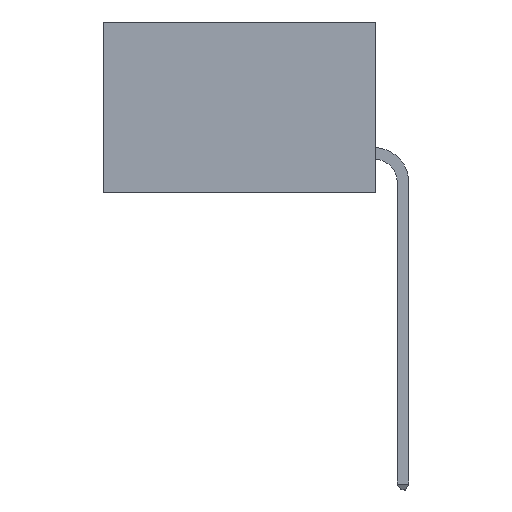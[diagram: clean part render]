
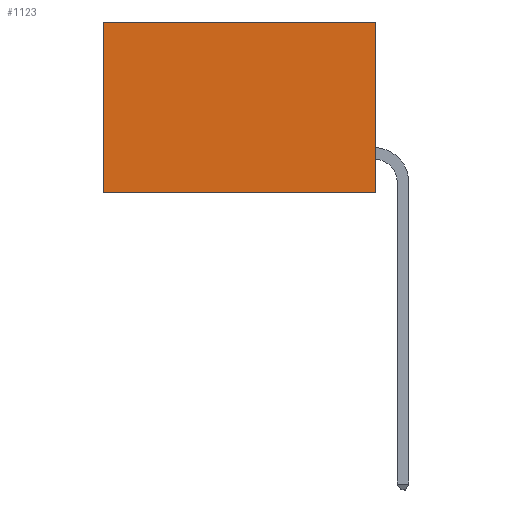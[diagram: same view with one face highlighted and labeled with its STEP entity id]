
A CAD part, left-side view. The second image highlights one B-rep face of the part: STEP entity #1123.
In plain terms, the highlighted planar face has unit normal (-1, 0, 0).
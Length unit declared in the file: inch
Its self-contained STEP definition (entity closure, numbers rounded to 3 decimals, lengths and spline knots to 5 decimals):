
#225 = CARTESIAN_POINT ( 'NONE',  ( 0.277, 0., -0.37 ) ) ;
#475 = VECTOR ( 'NONE', #12674, 39.37008 ) ;
#764 = AXIS2_PLACEMENT_3D ( 'NONE', #2841, #3631, #5499 ) ;
#955 = DIRECTION ( 'NONE',  ( 0., 1., 0. ) ) ;
#1123 = ADVANCED_FACE ( 'NONE', ( #13194 ), #10374, .F. ) ;
#1459 = VERTEX_POINT ( 'NONE', #225 ) ;
#1696 = VECTOR ( 'NONE', #955, 39.37008 ) ;
#2172 = EDGE_CURVE ( 'NONE', #10078, #1459, #9218, .T. ) ;
#2841 = CARTESIAN_POINT ( 'NONE',  ( 0.277, 0., -0.37 ) ) ;
#3599 = ORIENTED_EDGE ( 'NONE', *, *, #5665, .T. ) ;
#3601 = CARTESIAN_POINT ( 'NONE',  ( 0.277, 0., -0.37 ) ) ;
#3631 = DIRECTION ( 'NONE',  ( 1., 0., 0. ) ) ;
#3669 = ORIENTED_EDGE ( 'NONE', *, *, #4193, .F. ) ;
#3765 = ORIENTED_EDGE ( 'NONE', *, *, #2172, .F. ) ;
#3776 = ORIENTED_EDGE ( 'NONE', *, *, #13361, .T. ) ;
#4193 = EDGE_CURVE ( 'NONE', #1459, #6478, #6012, .T. ) ;
#5122 = VECTOR ( 'NONE', #7197, 39.37008 ) ;
#5499 = DIRECTION ( 'NONE',  ( 0., 0., -1. ) ) ;
#5665 = EDGE_CURVE ( 'NONE', #6463, #6478, #8031, .T. ) ;
#6012 = LINE ( 'NONE', #3601, #11280 ) ;
#6325 = CARTESIAN_POINT ( 'NONE',  ( 0.277, 0.59, -0.37 ) ) ;
#6463 = VERTEX_POINT ( 'NONE', #6680 ) ;
#6478 = VERTEX_POINT ( 'NONE', #6325 ) ;
#6680 = CARTESIAN_POINT ( 'NONE',  ( 0.277, 0.59, 0. ) ) ;
#7028 = CARTESIAN_POINT ( 'NONE',  ( 0.277, 0., -0.37 ) ) ;
#7152 = CARTESIAN_POINT ( 'NONE',  ( 0.277, 0.59, -0.37 ) ) ;
#7197 = DIRECTION ( 'NONE',  ( 0., 0., -1. ) ) ;
#8031 = LINE ( 'NONE', #7152, #5122 ) ;
#9102 = CARTESIAN_POINT ( 'NONE',  ( 0.277, 0., 0. ) ) ;
#9211 = DIRECTION ( 'NONE',  ( 0., 1., 0. ) ) ;
#9218 = LINE ( 'NONE', #7028, #475 ) ;
#10078 = VERTEX_POINT ( 'NONE', #9102 ) ;
#10374 = PLANE ( 'NONE',  #764 ) ;
#11280 = VECTOR ( 'NONE', #9211, 39.37008 ) ;
#12674 = DIRECTION ( 'NONE',  ( 0., 0., -1. ) ) ;
#12914 = EDGE_LOOP ( 'NONE', ( #3599, #3669, #3765, #3776 ) ) ;
#13047 = LINE ( 'NONE', #13704, #1696 ) ;
#13194 = FACE_OUTER_BOUND ( 'NONE', #12914, .T. ) ;
#13361 = EDGE_CURVE ( 'NONE', #10078, #6463, #13047, .T. ) ;
#13704 = CARTESIAN_POINT ( 'NONE',  ( 0.277, 0., 0. ) ) ;
